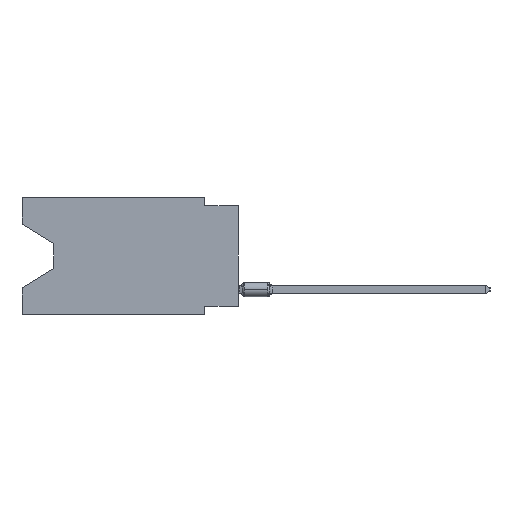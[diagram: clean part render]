
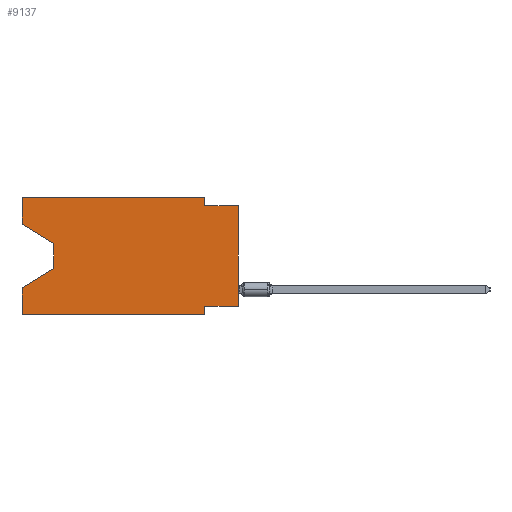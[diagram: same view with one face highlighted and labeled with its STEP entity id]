
A CAD part, left-side view. The second image highlights one B-rep face of the part: STEP entity #9137.
In plain terms, the highlighted planar face has unit normal (-1, 0, 0).
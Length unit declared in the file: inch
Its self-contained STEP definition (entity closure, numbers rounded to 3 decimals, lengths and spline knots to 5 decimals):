
#103 = VECTOR ( 'NONE', #10781, 39.37008 ) ;
#135 = ORIENTED_EDGE ( 'NONE', *, *, #2484, .T. ) ;
#342 = LINE ( 'NONE', #11803, #103 ) ;
#395 = DIRECTION ( 'NONE',  ( 0., 0., -1. ) ) ;
#403 = EDGE_CURVE ( 'NONE', #3476, #1875, #2060, .T. ) ;
#754 = CARTESIAN_POINT ( 'NONE',  ( 0., 0.645, 0. ) ) ;
#827 = ORIENTED_EDGE ( 'NONE', *, *, #3606, .T. ) ;
#1458 = VECTOR ( 'NONE', #7581, 39.37008 ) ;
#1580 = VECTOR ( 'NONE', #1768, 39.37008 ) ;
#1633 = CARTESIAN_POINT ( 'NONE',  ( 0., 0.55, -0.212 ) ) ;
#1645 = CARTESIAN_POINT ( 'NONE',  ( 0., 0.645, 0. ) ) ;
#1657 = CARTESIAN_POINT ( 'NONE',  ( 0., 0.1, -0.325 ) ) ;
#1752 = CARTESIAN_POINT ( 'NONE',  ( 0., 0.1, -0.025 ) ) ;
#1768 = DIRECTION ( 'NONE',  ( 0., 0., 1. ) ) ;
#1875 = VERTEX_POINT ( 'NONE', #9945 ) ;
#1987 = DIRECTION ( 'NONE',  ( 0., 0.855, -0.519 ) ) ;
#2060 = LINE ( 'NONE', #11366, #13186 ) ;
#2135 = CARTESIAN_POINT ( 'NONE',  ( 0., 0.645, -0.35 ) ) ;
#2164 = CARTESIAN_POINT ( 'NONE',  ( 0., 0.1, 0. ) ) ;
#2268 = VECTOR ( 'NONE', #5551, 39.37008 ) ;
#2370 = CARTESIAN_POINT ( 'NONE',  ( 0., 0.55, -0.138 ) ) ;
#2377 = VECTOR ( 'NONE', #395, 39.37008 ) ;
#2464 = CARTESIAN_POINT ( 'NONE',  ( 0., 0., -0.325 ) ) ;
#2484 = EDGE_CURVE ( 'NONE', #12332, #3476, #3274, .T. ) ;
#2497 = CARTESIAN_POINT ( 'NONE',  ( 0., 0., -0.025 ) ) ;
#2532 = LINE ( 'NONE', #6858, #2268 ) ;
#2560 = EDGE_CURVE ( 'NONE', #6758, #12332, #6761, .T. ) ;
#2680 = ORIENTED_EDGE ( 'NONE', *, *, #3843, .F. ) ;
#3058 = LINE ( 'NONE', #8399, #6108 ) ;
#3097 = EDGE_CURVE ( 'NONE', #8818, #8127, #11104, .T. ) ;
#3274 = LINE ( 'NONE', #2370, #1458 ) ;
#3476 = VERTEX_POINT ( 'NONE', #1633 ) ;
#3606 = EDGE_CURVE ( 'NONE', #10770, #6318, #3058, .T. ) ;
#3611 = DIRECTION ( 'NONE',  ( 0., -0.855, -0.519 ) ) ;
#3662 = CARTESIAN_POINT ( 'NONE',  ( 0., 0.1, -0.35 ) ) ;
#3755 = CARTESIAN_POINT ( 'NONE',  ( 0., 0.645, 0. ) ) ;
#3769 = ORIENTED_EDGE ( 'NONE', *, *, #2560, .T. ) ;
#3843 = EDGE_CURVE ( 'NONE', #8604, #6719, #5510, .T. ) ;
#3881 = DIRECTION ( 'NONE',  ( 0., -1., 0. ) ) ;
#3958 = ORIENTED_EDGE ( 'NONE', *, *, #4043, .F. ) ;
#4043 = EDGE_CURVE ( 'NONE', #6719, #6318, #5855, .T. ) ;
#4055 = VERTEX_POINT ( 'NONE', #11112 ) ;
#4156 = CARTESIAN_POINT ( 'NONE',  ( 0., 0.1, -0.35 ) ) ;
#4259 = DIRECTION ( 'NONE',  ( 0., -1., 0. ) ) ;
#4455 = ORIENTED_EDGE ( 'NONE', *, *, #10695, .F. ) ;
#4821 = DIRECTION ( 'NONE',  ( 0., -1., 0. ) ) ;
#4822 = CARTESIAN_POINT ( 'NONE',  ( 0., 0.645, -0.08025 ) ) ;
#5343 = CARTESIAN_POINT ( 'NONE',  ( 0., 0.55, -0.138 ) ) ;
#5510 = LINE ( 'NONE', #2164, #2377 ) ;
#5551 = DIRECTION ( 'NONE',  ( 0., 0., 1. ) ) ;
#5645 = VERTEX_POINT ( 'NONE', #5983 ) ;
#5855 = LINE ( 'NONE', #2497, #8718 ) ;
#5983 = CARTESIAN_POINT ( 'NONE',  ( 0., 0.645, -0.35 ) ) ;
#6108 = VECTOR ( 'NONE', #7115, 39.37008 ) ;
#6274 = VECTOR ( 'NONE', #3611, 39.37008 ) ;
#6318 = VERTEX_POINT ( 'NONE', #10858 ) ;
#6719 = VERTEX_POINT ( 'NONE', #1752 ) ;
#6758 = VERTEX_POINT ( 'NONE', #4822 ) ;
#6761 = LINE ( 'NONE', #13028, #6274 ) ;
#6858 = CARTESIAN_POINT ( 'NONE',  ( 0., 0.645, 0. ) ) ;
#6982 = PLANE ( 'NONE',  #12696 ) ;
#7115 = DIRECTION ( 'NONE',  ( 0., 0., 1. ) ) ;
#7224 = ORIENTED_EDGE ( 'NONE', *, *, #12766, .F. ) ;
#7306 = EDGE_CURVE ( 'NONE', #5645, #8127, #11515, .T. ) ;
#7581 = DIRECTION ( 'NONE',  ( 0., 0., -1. ) ) ;
#7988 = LINE ( 'NONE', #754, #11866 ) ;
#8127 = VERTEX_POINT ( 'NONE', #4156 ) ;
#8321 = VECTOR ( 'NONE', #4259, 39.37008 ) ;
#8399 = CARTESIAN_POINT ( 'NONE',  ( 0., 0., 0. ) ) ;
#8604 = VERTEX_POINT ( 'NONE', #10878 ) ;
#8718 = VECTOR ( 'NONE', #4821, 39.37008 ) ;
#8818 = VERTEX_POINT ( 'NONE', #1657 ) ;
#9137 = ADVANCED_FACE ( 'NONE', ( #11281 ), #6982, .F. ) ;
#9945 = CARTESIAN_POINT ( 'NONE',  ( 0., 0.645, -0.26975 ) ) ;
#9979 = DIRECTION ( 'NONE',  ( 0., 0., -1. ) ) ;
#9989 = ORIENTED_EDGE ( 'NONE', *, *, #11269, .F. ) ;
#10055 = ORIENTED_EDGE ( 'NONE', *, *, #10824, .F. ) ;
#10225 = VECTOR ( 'NONE', #11927, 39.37008 ) ;
#10438 = ORIENTED_EDGE ( 'NONE', *, *, #7306, .T. ) ;
#10695 = EDGE_CURVE ( 'NONE', #4055, #8604, #7988, .T. ) ;
#10770 = VERTEX_POINT ( 'NONE', #2464 ) ;
#10781 = DIRECTION ( 'NONE',  ( 0., 1., 0. ) ) ;
#10824 = EDGE_CURVE ( 'NONE', #6758, #4055, #2532, .T. ) ;
#10858 = CARTESIAN_POINT ( 'NONE',  ( 0., 0., -0.025 ) ) ;
#10878 = CARTESIAN_POINT ( 'NONE',  ( 0., 0.1, 0. ) ) ;
#11069 = DIRECTION ( 'NONE',  ( 1., 0., 0. ) ) ;
#11104 = LINE ( 'NONE', #3662, #10225 ) ;
#11112 = CARTESIAN_POINT ( 'NONE',  ( 0., 0.645, 0. ) ) ;
#11269 = EDGE_CURVE ( 'NONE', #5645, #1875, #13242, .T. ) ;
#11281 = FACE_OUTER_BOUND ( 'NONE', #12203, .T. ) ;
#11366 = CARTESIAN_POINT ( 'NONE',  ( 0., 0.55, -0.212 ) ) ;
#11515 = LINE ( 'NONE', #2135, #8321 ) ;
#11803 = CARTESIAN_POINT ( 'NONE',  ( 0., 0., -0.325 ) ) ;
#11866 = VECTOR ( 'NONE', #3881, 39.37008 ) ;
#11927 = DIRECTION ( 'NONE',  ( 0., 0., -1. ) ) ;
#12203 = EDGE_LOOP ( 'NONE', ( #3769, #135, #12300, #9989, #10438, #12476, #7224, #827, #3958, #2680, #4455, #10055 ) ) ;
#12300 = ORIENTED_EDGE ( 'NONE', *, *, #403, .T. ) ;
#12332 = VERTEX_POINT ( 'NONE', #5343 ) ;
#12476 = ORIENTED_EDGE ( 'NONE', *, *, #3097, .F. ) ;
#12696 = AXIS2_PLACEMENT_3D ( 'NONE', #1645, #11069, #9979 ) ;
#12766 = EDGE_CURVE ( 'NONE', #10770, #8818, #342, .T. ) ;
#13028 = CARTESIAN_POINT ( 'NONE',  ( 0., 0.645, -0.08025 ) ) ;
#13186 = VECTOR ( 'NONE', #1987, 39.37008 ) ;
#13242 = LINE ( 'NONE', #3755, #1580 ) ;
